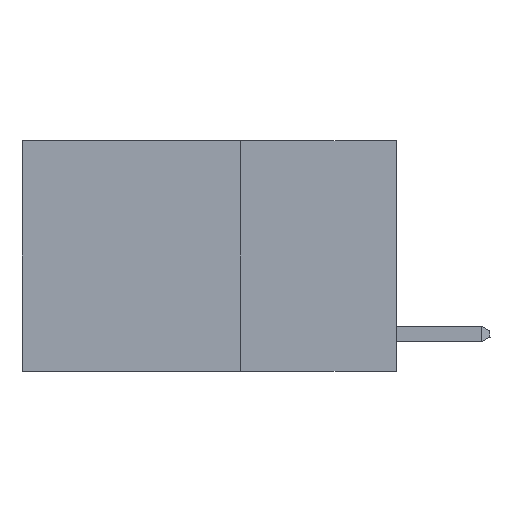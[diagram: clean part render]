
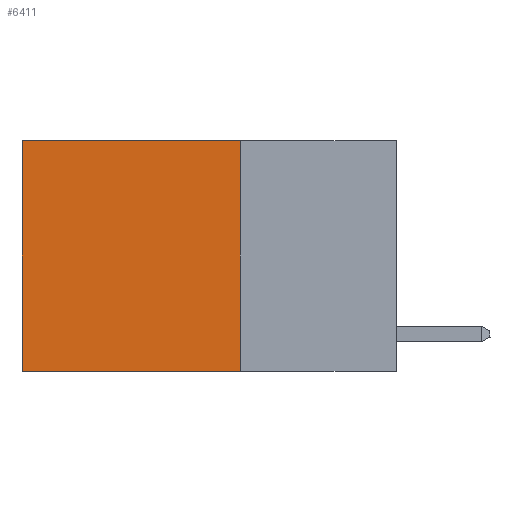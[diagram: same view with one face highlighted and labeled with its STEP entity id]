
A CAD part, left-side view. The second image highlights one B-rep face of the part: STEP entity #6411.
In plain terms, the highlighted planar face has unit normal (-1, 0, 0).
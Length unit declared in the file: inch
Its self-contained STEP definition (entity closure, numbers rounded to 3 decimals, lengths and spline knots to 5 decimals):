
#2200 = LINE ( 'NONE', #22728, #12746 ) ;
#3345 = ORIENTED_EDGE ( 'NONE', *, *, #8084, .T. ) ;
#3975 = LINE ( 'NONE', #25329, #25667 ) ;
#5237 = CARTESIAN_POINT ( 'NONE',  ( 0.2625, 0.25, 0. ) ) ;
#6411 = ADVANCED_FACE ( 'NONE', ( #13728 ), #26182, .F. ) ;
#7295 = EDGE_CURVE ( 'NONE', #16834, #12114, #2200, .T. ) ;
#7328 = DIRECTION ( 'NONE',  ( 0., 0., -1. ) ) ;
#7457 = VECTOR ( 'NONE', #22006, 39.37008 ) ;
#8084 = EDGE_CURVE ( 'NONE', #20011, #19515, #26506, .T. ) ;
#8437 = CARTESIAN_POINT ( 'NONE',  ( 0.2625, 0.6, -0.37 ) ) ;
#8494 = DIRECTION ( 'NONE',  ( 0., 0., -1. ) ) ;
#11234 = CARTESIAN_POINT ( 'NONE',  ( 0.2625, 0.25, -0.37 ) ) ;
#12114 = VERTEX_POINT ( 'NONE', #11234 ) ;
#12365 = CARTESIAN_POINT ( 'NONE',  ( 0.2625, 0.25, 0. ) ) ;
#12746 = VECTOR ( 'NONE', #8494, 39.37008 ) ;
#13728 = FACE_OUTER_BOUND ( 'NONE', #19931, .T. ) ;
#14942 = CARTESIAN_POINT ( 'NONE',  ( 0.2625, 0.6, 0. ) ) ;
#15007 = LINE ( 'NONE', #19862, #7457 ) ;
#15383 = ORIENTED_EDGE ( 'NONE', *, *, #7295, .F. ) ;
#16834 = VERTEX_POINT ( 'NONE', #12365 ) ;
#16941 = DIRECTION ( 'NONE',  ( 0., 1., 0. ) ) ;
#17064 = EDGE_CURVE ( 'NONE', #16834, #20011, #15007, .T. ) ;
#18914 = ORIENTED_EDGE ( 'NONE', *, *, #17064, .T. ) ;
#19515 = VERTEX_POINT ( 'NONE', #8437 ) ;
#19862 = CARTESIAN_POINT ( 'NONE',  ( 0.2625, 0.25, 0. ) ) ;
#19895 = DIRECTION ( 'NONE',  ( 1., 0., 0. ) ) ;
#19931 = EDGE_LOOP ( 'NONE', ( #3345, #24414, #15383, #18914 ) ) ;
#20011 = VERTEX_POINT ( 'NONE', #26772 ) ;
#20308 = AXIS2_PLACEMENT_3D ( 'NONE', #5237, #19895, #7328 ) ;
#20915 = VECTOR ( 'NONE', #23337, 39.37008 ) ;
#21550 = EDGE_CURVE ( 'NONE', #12114, #19515, #3975, .T. ) ;
#22006 = DIRECTION ( 'NONE',  ( 0., 1., 0. ) ) ;
#22728 = CARTESIAN_POINT ( 'NONE',  ( 0.2625, 0.25, 0. ) ) ;
#23337 = DIRECTION ( 'NONE',  ( 0., 0., -1. ) ) ;
#24414 = ORIENTED_EDGE ( 'NONE', *, *, #21550, .F. ) ;
#25329 = CARTESIAN_POINT ( 'NONE',  ( 0.2625, 0.25, -0.37 ) ) ;
#25667 = VECTOR ( 'NONE', #16941, 39.37008 ) ;
#26182 = PLANE ( 'NONE',  #20308 ) ;
#26506 = LINE ( 'NONE', #14942, #20915 ) ;
#26772 = CARTESIAN_POINT ( 'NONE',  ( 0.2625, 0.6, 0. ) ) ;
